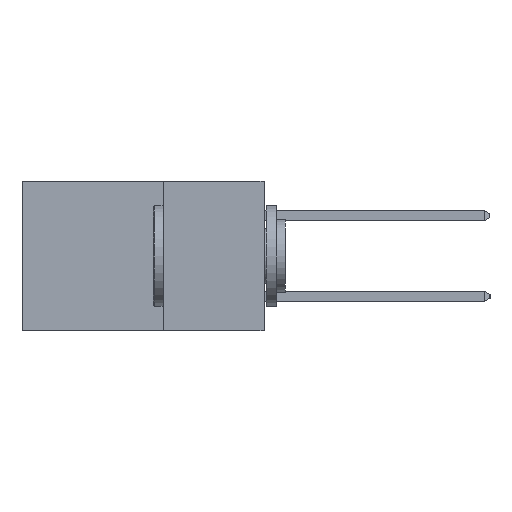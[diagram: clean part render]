
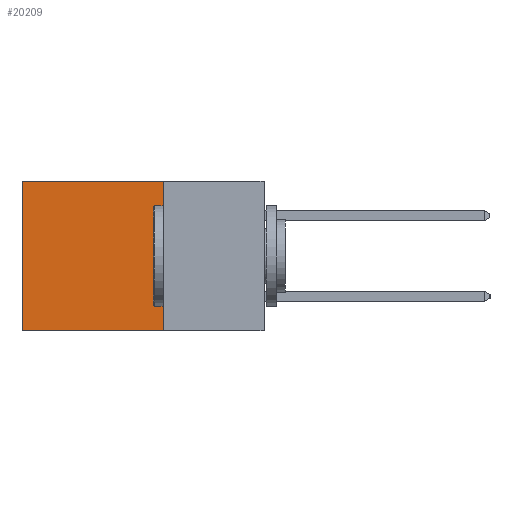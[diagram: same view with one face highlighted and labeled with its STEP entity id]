
A CAD part, left-side view. The second image highlights one B-rep face of the part: STEP entity #20209.
In plain terms, the highlighted planar face has unit normal (-1, 0, 0).
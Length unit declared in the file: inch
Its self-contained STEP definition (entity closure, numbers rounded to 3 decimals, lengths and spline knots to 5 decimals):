
#66 = CARTESIAN_POINT ( 'NONE',  ( 0.2615, 0.6, -0.37 ) ) ;
#2042 = EDGE_CURVE ( 'NONE', #11340, #15215, #11419, .T. ) ;
#2657 = AXIS2_PLACEMENT_3D ( 'NONE', #14836, #3439, #16714 ) ;
#3439 = DIRECTION ( 'NONE',  ( 1., 0., 0. ) ) ;
#3551 = CARTESIAN_POINT ( 'NONE',  ( 0.2615, 0.25, -0.37 ) ) ;
#5964 = DIRECTION ( 'NONE',  ( 0., 0., -1. ) ) ;
#6033 = VERTEX_POINT ( 'NONE', #16329 ) ;
#6601 = CARTESIAN_POINT ( 'NONE',  ( 0.2615, 0.25, 0. ) ) ;
#7649 = LINE ( 'NONE', #66, #22201 ) ;
#8498 = ORIENTED_EDGE ( 'NONE', *, *, #16220, .T. ) ;
#9244 = LINE ( 'NONE', #3551, #24368 ) ;
#10392 = ORIENTED_EDGE ( 'NONE', *, *, #21588, .F. ) ;
#10820 = VECTOR ( 'NONE', #21780, 39.37008 ) ;
#11223 = DIRECTION ( 'NONE',  ( 0., 1., 0. ) ) ;
#11340 = VERTEX_POINT ( 'NONE', #12164 ) ;
#11419 = LINE ( 'NONE', #6601, #10820 ) ;
#11658 = CARTESIAN_POINT ( 'NONE',  ( 0.2615, 0.6, 0. ) ) ;
#12164 = CARTESIAN_POINT ( 'NONE',  ( 0.2615, 0.25, 0. ) ) ;
#12204 = LINE ( 'NONE', #22965, #16642 ) ;
#12527 = EDGE_CURVE ( 'NONE', #11340, #6033, #12204, .T. ) ;
#13452 = ORIENTED_EDGE ( 'NONE', *, *, #2042, .T. ) ;
#14836 = CARTESIAN_POINT ( 'NONE',  ( 0.2615, 0.25, -0.37 ) ) ;
#15215 = VERTEX_POINT ( 'NONE', #11658 ) ;
#15794 = ORIENTED_EDGE ( 'NONE', *, *, #12527, .F. ) ;
#16220 = EDGE_CURVE ( 'NONE', #15215, #23622, #7649, .T. ) ;
#16329 = CARTESIAN_POINT ( 'NONE',  ( 0.2615, 0.25, -0.37 ) ) ;
#16637 = PLANE ( 'NONE',  #2657 ) ;
#16642 = VECTOR ( 'NONE', #5964, 39.37008 ) ;
#16714 = DIRECTION ( 'NONE',  ( 0., 0., -1. ) ) ;
#18545 = CARTESIAN_POINT ( 'NONE',  ( 0.2615, 0.6, -0.37 ) ) ;
#19012 = DIRECTION ( 'NONE',  ( 0., 0., -1. ) ) ;
#19368 = FACE_OUTER_BOUND ( 'NONE', #23743, .T. ) ;
#20209 = ADVANCED_FACE ( 'NONE', ( #19368 ), #16637, .F. ) ;
#21588 = EDGE_CURVE ( 'NONE', #6033, #23622, #9244, .T. ) ;
#21780 = DIRECTION ( 'NONE',  ( 0., 1., 0. ) ) ;
#22201 = VECTOR ( 'NONE', #19012, 39.37008 ) ;
#22965 = CARTESIAN_POINT ( 'NONE',  ( 0.2615, 0.25, -0.37 ) ) ;
#23622 = VERTEX_POINT ( 'NONE', #18545 ) ;
#23743 = EDGE_LOOP ( 'NONE', ( #8498, #10392, #15794, #13452 ) ) ;
#24368 = VECTOR ( 'NONE', #11223, 39.37008 ) ;
